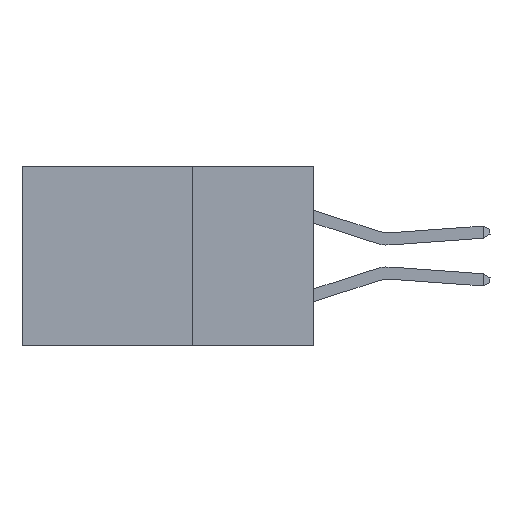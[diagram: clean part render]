
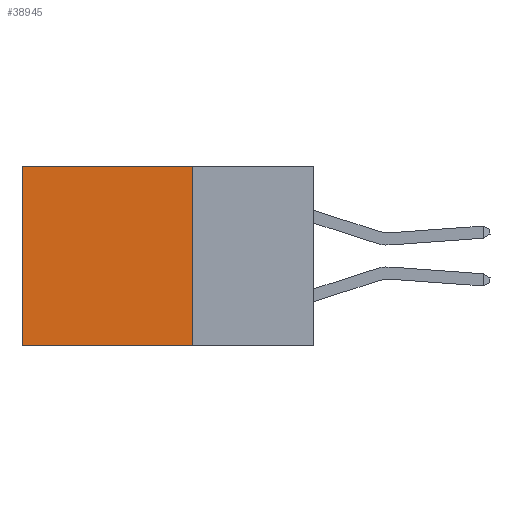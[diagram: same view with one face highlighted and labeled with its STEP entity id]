
A CAD part, left-side view. The second image highlights one B-rep face of the part: STEP entity #38945.
In plain terms, the highlighted planar face has unit normal (-1, 0, 0).
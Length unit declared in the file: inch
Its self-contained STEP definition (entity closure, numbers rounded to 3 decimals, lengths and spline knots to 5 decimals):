
#137 = DIRECTION ( 'NONE',  ( 0., 1., 0. ) ) ;
#1697 = LINE ( 'NONE', #19997, #29009 ) ;
#3925 = CARTESIAN_POINT ( 'NONE',  ( 0.2875, 0.25, -0.37 ) ) ;
#5159 = EDGE_LOOP ( 'NONE', ( #6451, #44751, #24512, #22080 ) ) ;
#5267 = CARTESIAN_POINT ( 'NONE',  ( 0.2875, 0.25, 0. ) ) ;
#6451 = ORIENTED_EDGE ( 'NONE', *, *, #30179, .T. ) ;
#7262 = CARTESIAN_POINT ( 'NONE',  ( 0.2875, 0.25, 0. ) ) ;
#9035 = AXIS2_PLACEMENT_3D ( 'NONE', #19998, #47707, #43542 ) ;
#9405 = VERTEX_POINT ( 'NONE', #40519 ) ;
#16451 = EDGE_CURVE ( 'NONE', #33173, #9405, #38802, .T. ) ;
#17136 = VECTOR ( 'NONE', #137, 39.37008 ) ;
#18496 = CARTESIAN_POINT ( 'NONE',  ( 0.2875, 0.25, -0.37 ) ) ;
#19997 = CARTESIAN_POINT ( 'NONE',  ( 0.2875, 0.6, 0. ) ) ;
#19998 = CARTESIAN_POINT ( 'NONE',  ( 0.2875, 0.25, 0. ) ) ;
#20207 = LINE ( 'NONE', #3925, #17136 ) ;
#22080 = ORIENTED_EDGE ( 'NONE', *, *, #16451, .T. ) ;
#23935 = DIRECTION ( 'NONE',  ( 0., 0., -1. ) ) ;
#24512 = ORIENTED_EDGE ( 'NONE', *, *, #50162, .F. ) ;
#28356 = PLANE ( 'NONE',  #9035 ) ;
#29009 = VECTOR ( 'NONE', #39914, 39.37008 ) ;
#29721 = VERTEX_POINT ( 'NONE', #41686 ) ;
#30179 = EDGE_CURVE ( 'NONE', #9405, #29721, #1697, .T. ) ;
#33173 = VERTEX_POINT ( 'NONE', #5267 ) ;
#38802 = LINE ( 'NONE', #7262, #42533 ) ;
#38945 = ADVANCED_FACE ( 'NONE', ( #40416 ), #28356, .F. ) ;
#39914 = DIRECTION ( 'NONE',  ( 0., 0., -1. ) ) ;
#40416 = FACE_OUTER_BOUND ( 'NONE', #5159, .T. ) ;
#40519 = CARTESIAN_POINT ( 'NONE',  ( 0.2875, 0.6, 0. ) ) ;
#41686 = CARTESIAN_POINT ( 'NONE',  ( 0.2875, 0.6, -0.37 ) ) ;
#42380 = VERTEX_POINT ( 'NONE', #18496 ) ;
#42533 = VECTOR ( 'NONE', #46594, 39.37008 ) ;
#43542 = DIRECTION ( 'NONE',  ( 0., 0., -1. ) ) ;
#43865 = VECTOR ( 'NONE', #23935, 39.37008 ) ;
#44143 = CARTESIAN_POINT ( 'NONE',  ( 0.2875, 0.25, 0. ) ) ;
#44466 = LINE ( 'NONE', #44143, #43865 ) ;
#44751 = ORIENTED_EDGE ( 'NONE', *, *, #50733, .F. ) ;
#46594 = DIRECTION ( 'NONE',  ( 0., 1., 0. ) ) ;
#47707 = DIRECTION ( 'NONE',  ( 1., 0., 0. ) ) ;
#50162 = EDGE_CURVE ( 'NONE', #33173, #42380, #44466, .T. ) ;
#50733 = EDGE_CURVE ( 'NONE', #42380, #29721, #20207, .T. ) ;
